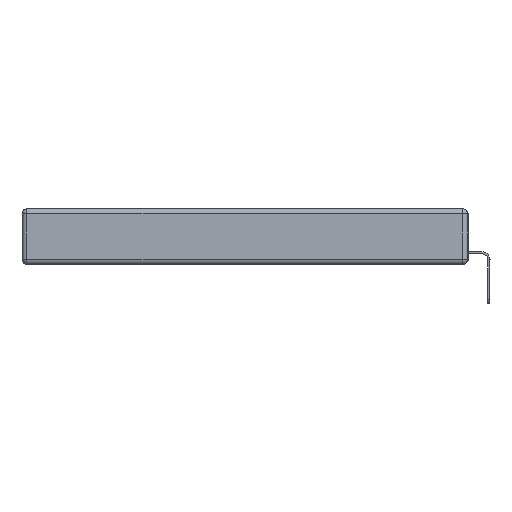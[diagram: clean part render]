
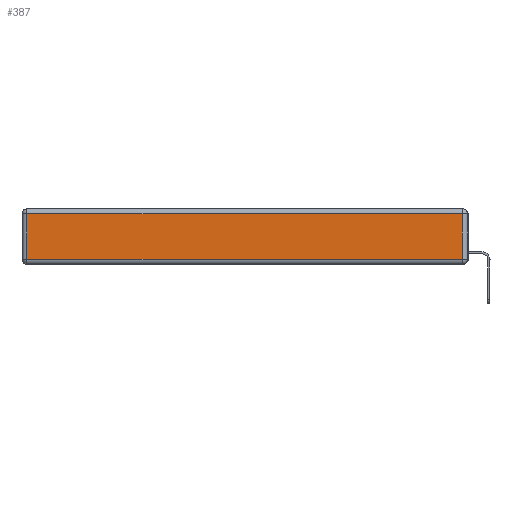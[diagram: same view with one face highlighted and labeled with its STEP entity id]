
A CAD part, left-side view. The second image highlights one B-rep face of the part: STEP entity #387.
In plain terms, the highlighted planar face has unit normal (-1, 0, 0).
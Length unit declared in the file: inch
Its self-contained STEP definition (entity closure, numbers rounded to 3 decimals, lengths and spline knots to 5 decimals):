
#52 = DIRECTION ( 'NONE',  ( 0., 0., 1. ) ) ;
#387 = ADVANCED_FACE ( 'NONE', ( #14157 ), #13071, .T. ) ;
#998 = CARTESIAN_POINT ( 'NONE',  ( 0., 0.03, -0.313 ) ) ;
#1168 = VECTOR ( 'NONE', #7446, 39.37008 ) ;
#1604 = EDGE_CURVE ( 'NONE', #8187, #7829, #13875, .T. ) ;
#2435 = VERTEX_POINT ( 'NONE', #5152 ) ;
#2648 = EDGE_CURVE ( 'NONE', #7829, #9192, #6702, .T. ) ;
#2989 = ORIENTED_EDGE ( 'NONE', *, *, #1604, .T. ) ;
#3726 = ORIENTED_EDGE ( 'NONE', *, *, #6595, .T. ) ;
#3855 = DIRECTION ( 'NONE',  ( 0., 0., 1. ) ) ;
#3982 = CARTESIAN_POINT ( 'NONE',  ( 0., 0.03, -0.343 ) ) ;
#4061 = VECTOR ( 'NONE', #11685, 39.37008 ) ;
#4279 = CARTESIAN_POINT ( 'NONE',  ( 0., 0., -0.343 ) ) ;
#4465 = DIRECTION ( 'NONE',  ( 0., -1., 0. ) ) ;
#4683 = ORIENTED_EDGE ( 'NONE', *, *, #5061, .T. ) ;
#5061 = EDGE_CURVE ( 'NONE', #2435, #8187, #13102, .T. ) ;
#5152 = CARTESIAN_POINT ( 'NONE',  ( 0., 2.72, -0.03 ) ) ;
#5743 = DIRECTION ( 'NONE',  ( -1., 0., 0. ) ) ;
#6588 = LINE ( 'NONE', #19043, #4061 ) ;
#6595 = EDGE_CURVE ( 'NONE', #9192, #2435, #6588, .T. ) ;
#6702 = LINE ( 'NONE', #3982, #13149 ) ;
#6911 = CARTESIAN_POINT ( 'NONE',  ( 0., 0.03, -0.03 ) ) ;
#7096 = ORIENTED_EDGE ( 'NONE', *, *, #2648, .T. ) ;
#7390 = EDGE_LOOP ( 'NONE', ( #2989, #7096, #3726, #4683 ) ) ;
#7446 = DIRECTION ( 'NONE',  ( 0., 0., -1. ) ) ;
#7829 = VERTEX_POINT ( 'NONE', #998 ) ;
#8187 = VERTEX_POINT ( 'NONE', #13761 ) ;
#8580 = VECTOR ( 'NONE', #4465, 39.37008 ) ;
#9192 = VERTEX_POINT ( 'NONE', #6911 ) ;
#11685 = DIRECTION ( 'NONE',  ( 0., 1., 0. ) ) ;
#13071 = PLANE ( 'NONE',  #18513 ) ;
#13102 = LINE ( 'NONE', #13501, #1168 ) ;
#13149 = VECTOR ( 'NONE', #3855, 39.37008 ) ;
#13501 = CARTESIAN_POINT ( 'NONE',  ( 0., 2.72, -0.343 ) ) ;
#13761 = CARTESIAN_POINT ( 'NONE',  ( 0., 2.72, -0.313 ) ) ;
#13875 = LINE ( 'NONE', #16246, #8580 ) ;
#14157 = FACE_OUTER_BOUND ( 'NONE', #7390, .T. ) ;
#16246 = CARTESIAN_POINT ( 'NONE',  ( 0., 0., -0.313 ) ) ;
#18513 = AXIS2_PLACEMENT_3D ( 'NONE', #4279, #5743, #52 ) ;
#19043 = CARTESIAN_POINT ( 'NONE',  ( 0., 2.75, -0.03 ) ) ;
